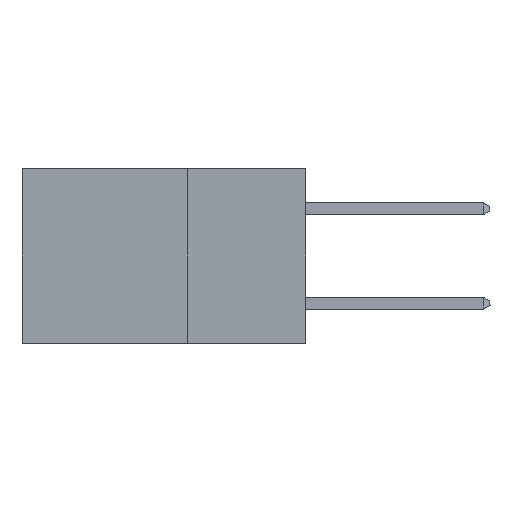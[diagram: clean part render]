
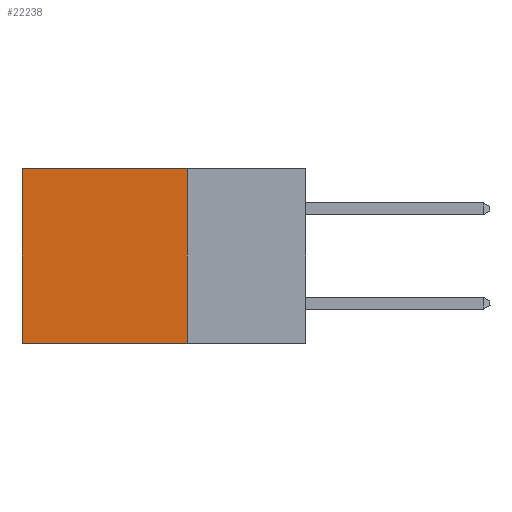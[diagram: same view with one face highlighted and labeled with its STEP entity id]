
A CAD part, left-side view. The second image highlights one B-rep face of the part: STEP entity #22238.
In plain terms, the highlighted planar face has unit normal (-1, 0, 0).
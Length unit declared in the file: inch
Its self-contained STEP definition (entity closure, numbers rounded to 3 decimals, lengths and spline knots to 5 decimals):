
#1206 = DIRECTION ( 'NONE',  ( 0., 1., 0. ) ) ;
#1943 = VECTOR ( 'NONE', #10105, 39.37008 ) ;
#1998 = LINE ( 'NONE', #19050, #16844 ) ;
#2260 = EDGE_CURVE ( 'NONE', #14612, #3342, #21328, .T. ) ;
#2351 = CARTESIAN_POINT ( 'NONE',  ( 0.298, 0.25, 0. ) ) ;
#2642 = EDGE_LOOP ( 'NONE', ( #9155, #7817, #3756, #13652 ) ) ;
#3342 = VERTEX_POINT ( 'NONE', #13611 ) ;
#3756 = ORIENTED_EDGE ( 'NONE', *, *, #18476, .F. ) ;
#5239 = VERTEX_POINT ( 'NONE', #10213 ) ;
#5637 = DIRECTION ( 'NONE',  ( 0., 0., -1. ) ) ;
#6302 = VECTOR ( 'NONE', #1206, 39.37008 ) ;
#7604 = AXIS2_PLACEMENT_3D ( 'NONE', #13217, #17022, #5637 ) ;
#7787 = DIRECTION ( 'NONE',  ( 0., 0., -1. ) ) ;
#7817 = ORIENTED_EDGE ( 'NONE', *, *, #19366, .F. ) ;
#9155 = ORIENTED_EDGE ( 'NONE', *, *, #12997, .T. ) ;
#9728 = CARTESIAN_POINT ( 'NONE',  ( 0.298, 0.6, 0. ) ) ;
#10105 = DIRECTION ( 'NONE',  ( 0., 1., 0. ) ) ;
#10213 = CARTESIAN_POINT ( 'NONE',  ( 0.298, 0.6, -0.37 ) ) ;
#11955 = CARTESIAN_POINT ( 'NONE',  ( 0.298, 0.25, -0.37 ) ) ;
#11984 = FACE_OUTER_BOUND ( 'NONE', #2642, .T. ) ;
#12997 = EDGE_CURVE ( 'NONE', #3342, #5239, #20665, .T. ) ;
#13217 = CARTESIAN_POINT ( 'NONE',  ( 0.298, 0.25, 0. ) ) ;
#13611 = CARTESIAN_POINT ( 'NONE',  ( 0.298, 0.6, 0. ) ) ;
#13652 = ORIENTED_EDGE ( 'NONE', *, *, #2260, .T. ) ;
#14612 = VERTEX_POINT ( 'NONE', #17302 ) ;
#14800 = CARTESIAN_POINT ( 'NONE',  ( 0.298, 0.25, -0.37 ) ) ;
#15314 = DIRECTION ( 'NONE',  ( 0., 0., -1. ) ) ;
#16299 = VERTEX_POINT ( 'NONE', #14800 ) ;
#16844 = VECTOR ( 'NONE', #7787, 39.37008 ) ;
#17022 = DIRECTION ( 'NONE',  ( 1., 0., 0. ) ) ;
#17302 = CARTESIAN_POINT ( 'NONE',  ( 0.298, 0.25, 0. ) ) ;
#17384 = LINE ( 'NONE', #11955, #1943 ) ;
#18476 = EDGE_CURVE ( 'NONE', #14612, #16299, #1998, .T. ) ;
#18811 = PLANE ( 'NONE',  #7604 ) ;
#19050 = CARTESIAN_POINT ( 'NONE',  ( 0.298, 0.25, 0. ) ) ;
#19366 = EDGE_CURVE ( 'NONE', #16299, #5239, #17384, .T. ) ;
#20092 = VECTOR ( 'NONE', #15314, 39.37008 ) ;
#20665 = LINE ( 'NONE', #9728, #20092 ) ;
#21328 = LINE ( 'NONE', #2351, #6302 ) ;
#22238 = ADVANCED_FACE ( 'NONE', ( #11984 ), #18811, .F. ) ;
